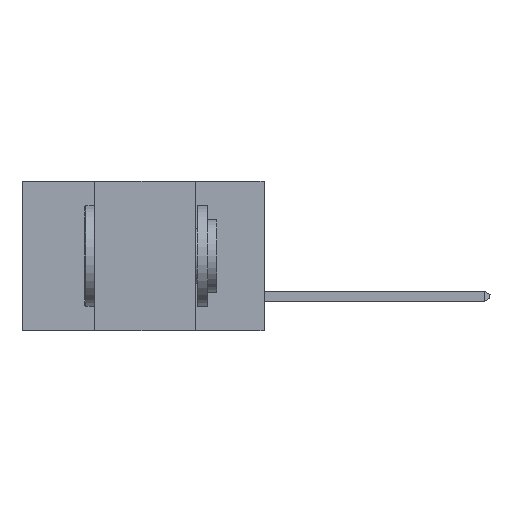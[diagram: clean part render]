
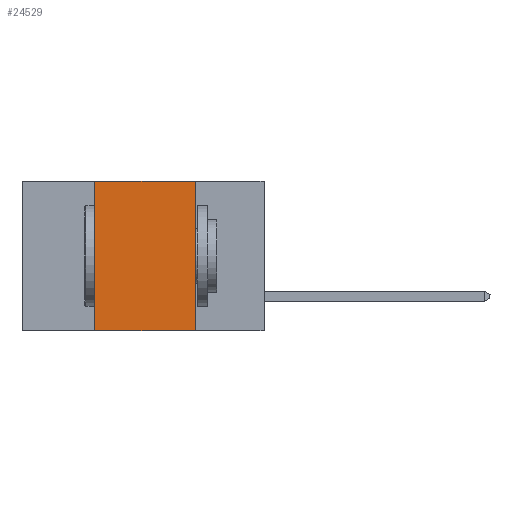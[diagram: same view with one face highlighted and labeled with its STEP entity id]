
A CAD part, left-side view. The second image highlights one B-rep face of the part: STEP entity #24529.
In plain terms, the highlighted planar face has unit normal (-1, 0, 0).
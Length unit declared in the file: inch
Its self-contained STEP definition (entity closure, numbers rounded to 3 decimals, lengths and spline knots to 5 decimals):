
#1367 = VERTEX_POINT ( 'NONE', #24357 ) ;
#3822 = CARTESIAN_POINT ( 'NONE',  ( 0., 0.6, 0. ) ) ;
#3950 = LINE ( 'NONE', #11650, #19941 ) ;
#4062 = VECTOR ( 'NONE', #23967, 39.37008 ) ;
#4814 = LINE ( 'NONE', #26172, #4062 ) ;
#6246 = EDGE_CURVE ( 'NONE', #9095, #1367, #10933, .T. ) ;
#7194 = VECTOR ( 'NONE', #29466, 39.37008 ) ;
#7424 = EDGE_CURVE ( 'NONE', #27172, #13321, #4814, .T. ) ;
#7587 = LINE ( 'NONE', #12515, #7194 ) ;
#9095 = VERTEX_POINT ( 'NONE', #24452 ) ;
#9239 = CARTESIAN_POINT ( 'NONE',  ( 0., 0.42, 0. ) ) ;
#9525 = AXIS2_PLACEMENT_3D ( 'NONE', #3822, #20744, #23049 ) ;
#10164 = CARTESIAN_POINT ( 'NONE',  ( 0., 0.17, 0. ) ) ;
#10560 = EDGE_CURVE ( 'NONE', #13321, #9095, #3950, .T. ) ;
#10933 = LINE ( 'NONE', #10164, #14759 ) ;
#11650 = CARTESIAN_POINT ( 'NONE',  ( 0., 0.6, 0. ) ) ;
#12515 = CARTESIAN_POINT ( 'NONE',  ( 0., 0.6, -0.37 ) ) ;
#12903 = FACE_OUTER_BOUND ( 'NONE', #30649, .T. ) ;
#13321 = VERTEX_POINT ( 'NONE', #9239 ) ;
#13479 = PLANE ( 'NONE',  #9525 ) ;
#13584 = EDGE_CURVE ( 'NONE', #27172, #1367, #7587, .T. ) ;
#14759 = VECTOR ( 'NONE', #17233, 39.37008 ) ;
#17233 = DIRECTION ( 'NONE',  ( 0., 0., -1. ) ) ;
#19941 = VECTOR ( 'NONE', #27118, 39.37008 ) ;
#20744 = DIRECTION ( 'NONE',  ( 1., 0., 0. ) ) ;
#20819 = ORIENTED_EDGE ( 'NONE', *, *, #7424, .F. ) ;
#21861 = CARTESIAN_POINT ( 'NONE',  ( 0., 0.42, -0.37 ) ) ;
#22818 = ORIENTED_EDGE ( 'NONE', *, *, #13584, .T. ) ;
#23049 = DIRECTION ( 'NONE',  ( 0., 0., -1. ) ) ;
#23967 = DIRECTION ( 'NONE',  ( 0., 0., 1. ) ) ;
#24357 = CARTESIAN_POINT ( 'NONE',  ( 0., 0.17, -0.37 ) ) ;
#24452 = CARTESIAN_POINT ( 'NONE',  ( 0., 0.17, 0. ) ) ;
#24529 = ADVANCED_FACE ( 'NONE', ( #12903 ), #13479, .F. ) ;
#26172 = CARTESIAN_POINT ( 'NONE',  ( 0., 0.42, 0. ) ) ;
#27118 = DIRECTION ( 'NONE',  ( 0., -1., 0. ) ) ;
#27172 = VERTEX_POINT ( 'NONE', #21861 ) ;
#29161 = ORIENTED_EDGE ( 'NONE', *, *, #10560, .F. ) ;
#29466 = DIRECTION ( 'NONE',  ( 0., -1., 0. ) ) ;
#30649 = EDGE_LOOP ( 'NONE', ( #31391, #29161, #20819, #22818 ) ) ;
#31391 = ORIENTED_EDGE ( 'NONE', *, *, #6246, .F. ) ;
